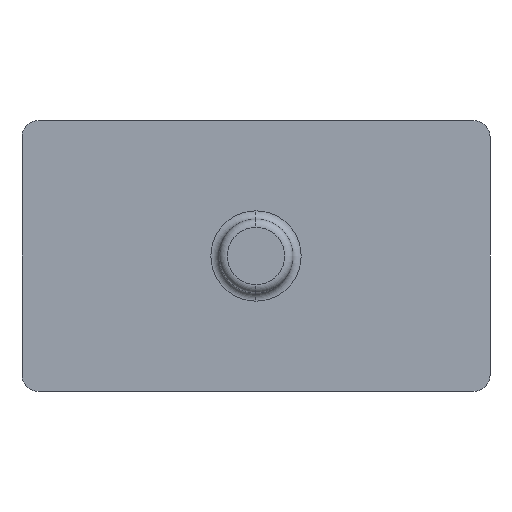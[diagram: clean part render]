
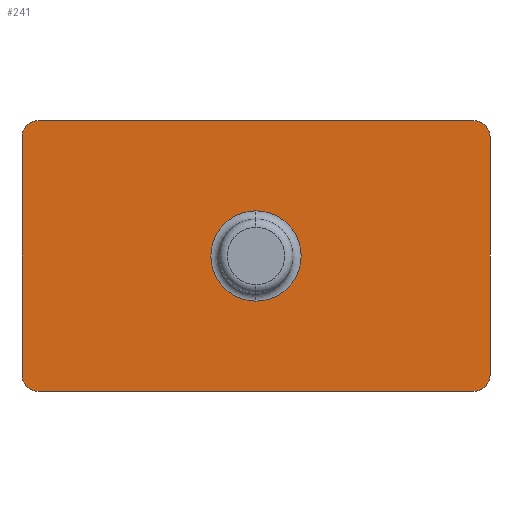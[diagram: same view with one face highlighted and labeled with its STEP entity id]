
A CAD part, front view. The second image highlights one B-rep face of the part: STEP entity #241.
In plain terms, the highlighted planar face has unit normal (0, -1, 0).
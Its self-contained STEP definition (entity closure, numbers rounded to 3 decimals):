
#11 = VECTOR ( 'NONE', #229, 1000. ) ;
#16 = DIRECTION ( 'NONE',  ( 0., 0., 1. ) ) ;
#28 = VERTEX_POINT ( 'NONE', #122 ) ;
#29 = EDGE_CURVE ( 'NONE', #130, #28, #328, .T. ) ;
#36 = CARTESIAN_POINT ( 'NONE',  ( -14.25, 0., -7.25 ) ) ;
#37 = DIRECTION ( 'NONE',  ( 0., 1., 0. ) ) ;
#39 = DIRECTION ( 'NONE',  ( 0., 0., 1. ) ) ;
#57 = CIRCLE ( 'NONE', #248, 1. ) ;
#58 = ORIENTED_EDGE ( 'NONE', *, *, #242, .T. ) ;
#77 = CARTESIAN_POINT ( 'NONE',  ( 13.25, 0., -8.25 ) ) ;
#80 = VECTOR ( 'NONE', #124, 1000. ) ;
#92 = ORIENTED_EDGE ( 'NONE', *, *, #113, .T. ) ;
#95 = CARTESIAN_POINT ( 'NONE',  ( -13.25, 0., 8.25 ) ) ;
#98 = CARTESIAN_POINT ( 'NONE',  ( 13.25, 0., -7.25 ) ) ;
#99 = CARTESIAN_POINT ( 'NONE',  ( 14.25, 0., -7.25 ) ) ;
#105 = ORIENTED_EDGE ( 'NONE', *, *, #29, .T. ) ;
#113 = EDGE_CURVE ( 'NONE', #192, #313, #365, .T. ) ;
#114 = LINE ( 'NONE', #221, #336 ) ;
#120 = DIRECTION ( 'NONE',  ( 0., -1., 0. ) ) ;
#122 = CARTESIAN_POINT ( 'NONE',  ( 0., 0., -2.75 ) ) ;
#124 = DIRECTION ( 'NONE',  ( 1., 0., 0. ) ) ;
#130 = VERTEX_POINT ( 'NONE', #205 ) ;
#134 = AXIS2_PLACEMENT_3D ( 'NONE', #366, #120, #406 ) ;
#139 = DIRECTION ( 'NONE',  ( 0., 0., -1. ) ) ;
#140 = LINE ( 'NONE', #273, #329 ) ;
#143 = DIRECTION ( 'NONE',  ( 0., 0., 1. ) ) ;
#144 = EDGE_LOOP ( 'NONE', ( #480, #58, #387, #491, #368, #92, #432, #470 ) ) ;
#147 = EDGE_CURVE ( 'NONE', #439, #301, #524, .T. ) ;
#162 = CARTESIAN_POINT ( 'NONE',  ( -14.25, 0., 0. ) ) ;
#164 = CARTESIAN_POINT ( 'NONE',  ( 0., 0., -8.25 ) ) ;
#174 = CARTESIAN_POINT ( 'NONE',  ( 13.25, 0., 7.25 ) ) ;
#187 = DIRECTION ( 'NONE',  ( 1., 0., 0. ) ) ;
#192 = VERTEX_POINT ( 'NONE', #36 ) ;
#196 = LINE ( 'NONE', #164, #80 ) ;
#197 = EDGE_CURVE ( 'NONE', #313, #204, #196, .T. ) ;
#201 = AXIS2_PLACEMENT_3D ( 'NONE', #302, #297, #289 ) ;
#204 = VERTEX_POINT ( 'NONE', #77 ) ;
#205 = CARTESIAN_POINT ( 'NONE',  ( 0., 0., 2.75 ) ) ;
#211 = DIRECTION ( 'NONE',  ( 0., 0., 1. ) ) ;
#213 = CARTESIAN_POINT ( 'NONE',  ( -13.25, 0., -8.25 ) ) ;
#216 = VERTEX_POINT ( 'NONE', #370 ) ;
#221 = CARTESIAN_POINT ( 'NONE',  ( 14.25, 0., 0. ) ) ;
#229 = DIRECTION ( 'NONE',  ( 0., 0., -1. ) ) ;
#241 = ADVANCED_FACE ( 'NONE', ( #490, #290 ), #294, .F. ) ;
#242 = EDGE_CURVE ( 'NONE', #216, #350, #57, .T. ) ;
#247 = DIRECTION ( 'NONE',  ( 0., -1., 0. ) ) ;
#248 = AXIS2_PLACEMENT_3D ( 'NONE', #174, #447, #211 ) ;
#269 = DIRECTION ( 'NONE',  ( 0., 1., 0. ) ) ;
#273 = CARTESIAN_POINT ( 'NONE',  ( 0., 0., 8.25 ) ) ;
#289 = DIRECTION ( 'NONE',  ( 0., 0., 1. ) ) ;
#290 = FACE_OUTER_BOUND ( 'NONE', #144, .T. ) ;
#292 = EDGE_LOOP ( 'NONE', ( #105, #452 ) ) ;
#294 = PLANE ( 'NONE',  #325 ) ;
#297 = DIRECTION ( 'NONE',  ( 0., 1., 0. ) ) ;
#301 = VERTEX_POINT ( 'NONE', #525 ) ;
#302 = CARTESIAN_POINT ( 'NONE',  ( 0., 0., 0. ) ) ;
#313 = VERTEX_POINT ( 'NONE', #213 ) ;
#325 = AXIS2_PLACEMENT_3D ( 'NONE', #489, #37, #39 ) ;
#328 = CIRCLE ( 'NONE', #201, 2.75 ) ;
#329 = VECTOR ( 'NONE', #187, 1000. ) ;
#336 = VECTOR ( 'NONE', #139, 1000. ) ;
#350 = VERTEX_POINT ( 'NONE', #455 ) ;
#356 = CIRCLE ( 'NONE', #467, 2.75 ) ;
#365 = CIRCLE ( 'NONE', #441, 1. ) ;
#366 = CARTESIAN_POINT ( 'NONE',  ( -13.25, 0., 7.25 ) ) ;
#368 = ORIENTED_EDGE ( 'NONE', *, *, #488, .T. ) ;
#370 = CARTESIAN_POINT ( 'NONE',  ( 14.25, 0., 7.25 ) ) ;
#387 = ORIENTED_EDGE ( 'NONE', *, *, #508, .F. ) ;
#388 = DIRECTION ( 'NONE',  ( 0., -1., 0. ) ) ;
#400 = EDGE_CURVE ( 'NONE', #216, #518, #114, .T. ) ;
#406 = DIRECTION ( 'NONE',  ( 0., 0., 1. ) ) ;
#432 = ORIENTED_EDGE ( 'NONE', *, *, #197, .T. ) ;
#436 = EDGE_CURVE ( 'NONE', #28, #130, #356, .T. ) ;
#439 = VERTEX_POINT ( 'NONE', #95 ) ;
#441 = AXIS2_PLACEMENT_3D ( 'NONE', #482, #247, #520 ) ;
#444 = LINE ( 'NONE', #162, #11 ) ;
#447 = DIRECTION ( 'NONE',  ( 0., -1., 0. ) ) ;
#449 = EDGE_CURVE ( 'NONE', #204, #518, #460, .T. ) ;
#452 = ORIENTED_EDGE ( 'NONE', *, *, #436, .T. ) ;
#455 = CARTESIAN_POINT ( 'NONE',  ( 13.25, 0., 8.25 ) ) ;
#460 = CIRCLE ( 'NONE', #516, 1. ) ;
#467 = AXIS2_PLACEMENT_3D ( 'NONE', #505, #269, #16 ) ;
#470 = ORIENTED_EDGE ( 'NONE', *, *, #449, .T. ) ;
#480 = ORIENTED_EDGE ( 'NONE', *, *, #400, .F. ) ;
#482 = CARTESIAN_POINT ( 'NONE',  ( -13.25, 0., -7.25 ) ) ;
#488 = EDGE_CURVE ( 'NONE', #301, #192, #444, .T. ) ;
#489 = CARTESIAN_POINT ( 'NONE',  ( 0., 0., 0. ) ) ;
#490 = FACE_BOUND ( 'NONE', #292, .T. ) ;
#491 = ORIENTED_EDGE ( 'NONE', *, *, #147, .T. ) ;
#505 = CARTESIAN_POINT ( 'NONE',  ( 0., 0., 0. ) ) ;
#508 = EDGE_CURVE ( 'NONE', #439, #350, #140, .T. ) ;
#516 = AXIS2_PLACEMENT_3D ( 'NONE', #98, #388, #143 ) ;
#518 = VERTEX_POINT ( 'NONE', #99 ) ;
#520 = DIRECTION ( 'NONE',  ( 0., 0., 1. ) ) ;
#524 = CIRCLE ( 'NONE', #134, 1. ) ;
#525 = CARTESIAN_POINT ( 'NONE',  ( -14.25, 0., 7.25 ) ) ;
